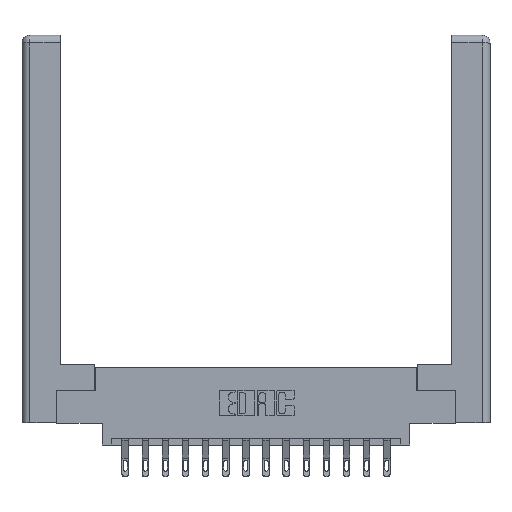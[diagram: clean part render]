
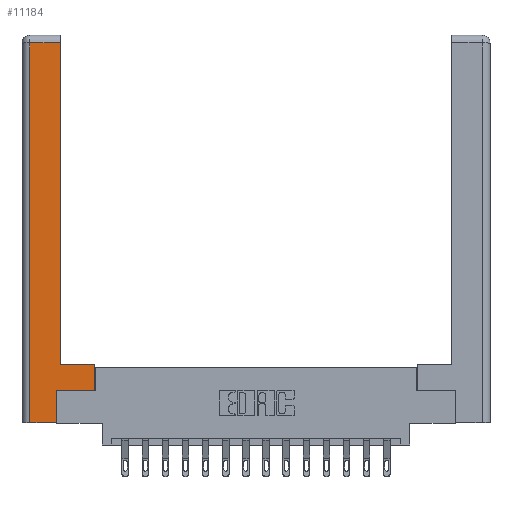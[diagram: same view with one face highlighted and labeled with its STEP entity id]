
A CAD part, top view. The second image highlights one B-rep face of the part: STEP entity #11184.
In plain terms, the highlighted planar face has unit normal (0, 0, 1).
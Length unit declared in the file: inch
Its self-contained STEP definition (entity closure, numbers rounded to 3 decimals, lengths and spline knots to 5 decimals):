
#552 = CARTESIAN_POINT ( 'NONE',  ( 0.295, 0.45, 0. ) ) ;
#1142 = EDGE_CURVE ( 'NONE', #11666, #14959, #1875, .T. ) ;
#1268 = ORIENTED_EDGE ( 'NONE', *, *, #12704, .T. ) ;
#1291 = VECTOR ( 'NONE', #3183, 39.37008 ) ;
#1651 = CARTESIAN_POINT ( 'NONE',  ( 0.565, 0.245, 0. ) ) ;
#1875 = LINE ( 'NONE', #5160, #5099 ) ;
#2036 = CARTESIAN_POINT ( 'NONE',  ( 0.295, 2.94, 0. ) ) ;
#2533 = ORIENTED_EDGE ( 'NONE', *, *, #7628, .T. ) ;
#2602 = DIRECTION ( 'NONE',  ( -1., 0., 0. ) ) ;
#2912 = CARTESIAN_POINT ( 'NONE',  ( 0.565, 0.245, 0. ) ) ;
#3040 = CARTESIAN_POINT ( 'NONE',  ( 0.265, 0.245, 0. ) ) ;
#3128 = VECTOR ( 'NONE', #7063, 39.37008 ) ;
#3144 = EDGE_LOOP ( 'NONE', ( #12483, #9878, #3749, #3264, #1268, #15756, #7978, #2533 ) ) ;
#3183 = DIRECTION ( 'NONE',  ( -1., 0., 0. ) ) ;
#3264 = ORIENTED_EDGE ( 'NONE', *, *, #13940, .T. ) ;
#3396 = VECTOR ( 'NONE', #11382, 39.37008 ) ;
#3702 = VERTEX_POINT ( 'NONE', #2036 ) ;
#3749 = ORIENTED_EDGE ( 'NONE', *, *, #7011, .T. ) ;
#4077 = VECTOR ( 'NONE', #12628, 39.37008 ) ;
#4899 = LINE ( 'NONE', #6238, #3396 ) ;
#5046 = CARTESIAN_POINT ( 'NONE',  ( 0., 0., 0. ) ) ;
#5099 = VECTOR ( 'NONE', #17144, 39.37008 ) ;
#5160 = CARTESIAN_POINT ( 'NONE',  ( 0.565, 0.45, 0. ) ) ;
#5796 = CARTESIAN_POINT ( 'NONE',  ( 0.0615, 0., 0. ) ) ;
#6238 = CARTESIAN_POINT ( 'NONE',  ( 0.295, 3., 0. ) ) ;
#6969 = CARTESIAN_POINT ( 'NONE',  ( 0.265, 0., 0. ) ) ;
#7011 = EDGE_CURVE ( 'NONE', #14189, #13550, #15596, .T. ) ;
#7063 = DIRECTION ( 'NONE',  ( 1., 0., 0. ) ) ;
#7549 = CARTESIAN_POINT ( 'NONE',  ( 0.565, 0.45, 0. ) ) ;
#7559 = CARTESIAN_POINT ( 'NONE',  ( 0.0615, 0., 0. ) ) ;
#7567 = CARTESIAN_POINT ( 'NONE',  ( 0.0615, 2.94, 0. ) ) ;
#7628 = EDGE_CURVE ( 'NONE', #14959, #14913, #8642, .T. ) ;
#7929 = LINE ( 'NONE', #11105, #11267 ) ;
#7978 = ORIENTED_EDGE ( 'NONE', *, *, #1142, .T. ) ;
#8291 = VECTOR ( 'NONE', #10706, 39.37008 ) ;
#8314 = CARTESIAN_POINT ( 'NONE',  ( 0.295, 0.45, 0. ) ) ;
#8642 = LINE ( 'NONE', #8314, #1291 ) ;
#9458 = CARTESIAN_POINT ( 'NONE',  ( 0.0615, 2.94, 0. ) ) ;
#9878 = ORIENTED_EDGE ( 'NONE', *, *, #14450, .T. ) ;
#10536 = DIRECTION ( 'NONE',  ( -1., 0., 0. ) ) ;
#10706 = DIRECTION ( 'NONE',  ( 1., 0., 0. ) ) ;
#10820 = VECTOR ( 'NONE', #2602, 39.37008 ) ;
#11105 = CARTESIAN_POINT ( 'NONE',  ( 0.265, 0.245, 0. ) ) ;
#11184 = ADVANCED_FACE ( 'NONE', ( #14092 ), #12973, .F. ) ;
#11267 = VECTOR ( 'NONE', #16422, 39.37008 ) ;
#11382 = DIRECTION ( 'NONE',  ( 0., 1., 0. ) ) ;
#11581 = VERTEX_POINT ( 'NONE', #3040 ) ;
#11666 = VERTEX_POINT ( 'NONE', #1651 ) ;
#11701 = EDGE_CURVE ( 'NONE', #14913, #3702, #4899, .T. ) ;
#11848 = DIRECTION ( 'NONE',  ( 0., 0., -1. ) ) ;
#12483 = ORIENTED_EDGE ( 'NONE', *, *, #11701, .T. ) ;
#12628 = DIRECTION ( 'NONE',  ( 0., -1., 0. ) ) ;
#12704 = EDGE_CURVE ( 'NONE', #17240, #11581, #7929, .T. ) ;
#12739 = LINE ( 'NONE', #2912, #3128 ) ;
#12973 = PLANE ( 'NONE',  #14474 ) ;
#13226 = EDGE_CURVE ( 'NONE', #11581, #11666, #12739, .T. ) ;
#13374 = LINE ( 'NONE', #17420, #8291 ) ;
#13550 = VERTEX_POINT ( 'NONE', #7559 ) ;
#13940 = EDGE_CURVE ( 'NONE', #13550, #17240, #13374, .T. ) ;
#14092 = FACE_OUTER_BOUND ( 'NONE', #3144, .T. ) ;
#14189 = VERTEX_POINT ( 'NONE', #7567 ) ;
#14450 = EDGE_CURVE ( 'NONE', #3702, #14189, #14458, .T. ) ;
#14458 = LINE ( 'NONE', #9458, #10820 ) ;
#14474 = AXIS2_PLACEMENT_3D ( 'NONE', #5046, #11848, #10536 ) ;
#14913 = VERTEX_POINT ( 'NONE', #552 ) ;
#14959 = VERTEX_POINT ( 'NONE', #7549 ) ;
#15596 = LINE ( 'NONE', #5796, #4077 ) ;
#15756 = ORIENTED_EDGE ( 'NONE', *, *, #13226, .T. ) ;
#16422 = DIRECTION ( 'NONE',  ( 0., 1., 0. ) ) ;
#17144 = DIRECTION ( 'NONE',  ( 0., 1., 0. ) ) ;
#17240 = VERTEX_POINT ( 'NONE', #6969 ) ;
#17420 = CARTESIAN_POINT ( 'NONE',  ( 0.265, 0., 0. ) ) ;
